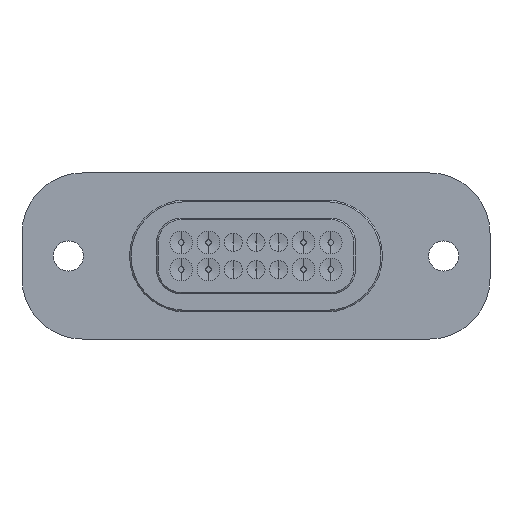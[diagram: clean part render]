
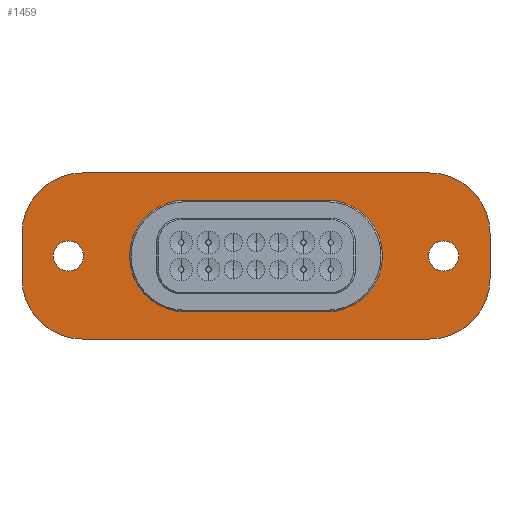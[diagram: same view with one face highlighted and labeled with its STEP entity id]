
A CAD part, front view. The second image highlights one B-rep face of the part: STEP entity #1459.
In plain terms, the highlighted planar face has unit normal (0, -1, 0).
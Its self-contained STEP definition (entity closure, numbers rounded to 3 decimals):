
#57 = DIRECTION ( 'NONE',  ( 0., 0., 1. ) ) ;
#124 = VERTEX_POINT ( 'NONE', #1518 ) ;
#156 = ORIENTED_EDGE ( 'NONE', *, *, #4023, .T. ) ;
#201 = CARTESIAN_POINT ( 'NONE',  ( 11.5, 0., 5.5 ) ) ;
#262 = DIRECTION ( 'NONE',  ( 0., 0., 1. ) ) ;
#278 = AXIS2_PLACEMENT_3D ( 'NONE', #2399, #5189, #822 ) ;
#284 = CARTESIAN_POINT ( 'NONE',  ( -15.5, 0., 1.5 ) ) ;
#300 = LINE ( 'NONE', #991, #3180 ) ;
#317 = EDGE_CURVE ( 'NONE', #6660, #124, #6042, .T. ) ;
#331 = VERTEX_POINT ( 'NONE', #3552 ) ;
#340 = EDGE_CURVE ( 'NONE', #4793, #2393, #2925, .T. ) ;
#360 = ORIENTED_EDGE ( 'NONE', *, *, #6810, .F. ) ;
#394 = ORIENTED_EDGE ( 'NONE', *, *, #2515, .F. ) ;
#575 = DIRECTION ( 'NONE',  ( 0., 0., 1. ) ) ;
#579 = CARTESIAN_POINT ( 'NONE',  ( 12.425, 0., -1. ) ) ;
#596 = DIRECTION ( 'NONE',  ( 0., 1., 0. ) ) ;
#610 = CIRCLE ( 'NONE', #1866, 4. ) ;
#712 = DIRECTION ( 'NONE',  ( 0., 0., -1. ) ) ;
#732 = DIRECTION ( 'NONE',  ( 1., 0., 0. ) ) ;
#759 = CARTESIAN_POINT ( 'NONE',  ( -4.675, 0., -3.7 ) ) ;
#817 = AXIS2_PLACEMENT_3D ( 'NONE', #6340, #1377, #262 ) ;
#818 = AXIS2_PLACEMENT_3D ( 'NONE', #2684, #4881, #575 ) ;
#822 = DIRECTION ( 'NONE',  ( 0., 0., 1. ) ) ;
#828 = EDGE_CURVE ( 'NONE', #3675, #5938, #7060, .T. ) ;
#859 = EDGE_CURVE ( 'NONE', #4183, #4793, #2325, .T. ) ;
#927 = ORIENTED_EDGE ( 'NONE', *, *, #3309, .F. ) ;
#945 = VERTEX_POINT ( 'NONE', #201 ) ;
#991 = CARTESIAN_POINT ( 'NONE',  ( -4.675, 0., 3.7 ) ) ;
#1001 = CARTESIAN_POINT ( 'NONE',  ( 4.675, 0., -3.7 ) ) ;
#1106 = DIRECTION ( 'NONE',  ( 0., -1., 0. ) ) ;
#1184 = VECTOR ( 'NONE', #2231, 1000. ) ;
#1231 = FACE_OUTER_BOUND ( 'NONE', #4790, .T. ) ;
#1261 = AXIS2_PLACEMENT_3D ( 'NONE', #5652, #4681, #5688 ) ;
#1334 = CARTESIAN_POINT ( 'NONE',  ( -15.5, 0., -1.5 ) ) ;
#1377 = DIRECTION ( 'NONE',  ( 0., -1., 0. ) ) ;
#1415 = ORIENTED_EDGE ( 'NONE', *, *, #2551, .F. ) ;
#1459 = ADVANCED_FACE ( 'NONE', ( #2762, #1695, #1231, #4932 ), #6038, .F. ) ;
#1518 = CARTESIAN_POINT ( 'NONE',  ( 12.425, 0., 1. ) ) ;
#1569 = VERTEX_POINT ( 'NONE', #3232 ) ;
#1596 = CIRCLE ( 'NONE', #1261, 4. ) ;
#1614 = CARTESIAN_POINT ( 'NONE',  ( -11.5, 0., 5.5 ) ) ;
#1695 = FACE_BOUND ( 'NONE', #6171, .T. ) ;
#1731 = DIRECTION ( 'NONE',  ( 0., 1., 0. ) ) ;
#1766 = ORIENTED_EDGE ( 'NONE', *, *, #3381, .F. ) ;
#1862 = ORIENTED_EDGE ( 'NONE', *, *, #6662, .F. ) ;
#1866 = AXIS2_PLACEMENT_3D ( 'NONE', #6739, #5154, #3391 ) ;
#1937 = CARTESIAN_POINT ( 'NONE',  ( -11.5, 0., 5.5 ) ) ;
#2052 = ORIENTED_EDGE ( 'NONE', *, *, #6228, .F. ) ;
#2111 = DIRECTION ( 'NONE',  ( -1., 0., 0. ) ) ;
#2172 = AXIS2_PLACEMENT_3D ( 'NONE', #6624, #1731, #2983 ) ;
#2215 = VECTOR ( 'NONE', #2111, 1000. ) ;
#2231 = DIRECTION ( 'NONE',  ( 0., 0., 1. ) ) ;
#2275 = CARTESIAN_POINT ( 'NONE',  ( -15.5, 0., -1.5 ) ) ;
#2325 = CIRCLE ( 'NONE', #5071, 3.7 ) ;
#2327 = CARTESIAN_POINT ( 'NONE',  ( 15.5, 0., 1.5 ) ) ;
#2393 = VERTEX_POINT ( 'NONE', #1001 ) ;
#2399 = CARTESIAN_POINT ( 'NONE',  ( 12.425, 0., 0. ) ) ;
#2489 = DIRECTION ( 'NONE',  ( 0., -1., 0. ) ) ;
#2515 = EDGE_CURVE ( 'NONE', #945, #3675, #7050, .T. ) ;
#2551 = EDGE_CURVE ( 'NONE', #6208, #6693, #610, .T. ) ;
#2578 = EDGE_LOOP ( 'NONE', ( #360, #6477 ) ) ;
#2632 = ORIENTED_EDGE ( 'NONE', *, *, #859, .F. ) ;
#2638 = VECTOR ( 'NONE', #2963, 1000. ) ;
#2660 = ORIENTED_EDGE ( 'NONE', *, *, #6914, .T. ) ;
#2684 = CARTESIAN_POINT ( 'NONE',  ( -12.425, 0., 0. ) ) ;
#2745 = DIRECTION ( 'NONE',  ( 0., 0., 1. ) ) ;
#2762 = FACE_BOUND ( 'NONE', #2578, .T. ) ;
#2779 = CARTESIAN_POINT ( 'NONE',  ( -4.675, 0., 3.7 ) ) ;
#2925 = LINE ( 'NONE', #6197, #2638 ) ;
#2963 = DIRECTION ( 'NONE',  ( 1., 0., 0. ) ) ;
#2983 = DIRECTION ( 'NONE',  ( 0., 0., 1. ) ) ;
#2987 = DIRECTION ( 'NONE',  ( 0., 0., -1. ) ) ;
#3180 = VECTOR ( 'NONE', #5865, 1000. ) ;
#3190 = DIRECTION ( 'NONE',  ( 0., 0., 1. ) ) ;
#3232 = CARTESIAN_POINT ( 'NONE',  ( -12.425, 0., -1. ) ) ;
#3309 = EDGE_CURVE ( 'NONE', #5938, #5661, #1596, .T. ) ;
#3373 = AXIS2_PLACEMENT_3D ( 'NONE', #5493, #596, #57 ) ;
#3381 = EDGE_CURVE ( 'NONE', #6693, #945, #6826, .T. ) ;
#3391 = DIRECTION ( 'NONE',  ( 0., 0., 1. ) ) ;
#3552 = CARTESIAN_POINT ( 'NONE',  ( -11.5, 0., -5.5 ) ) ;
#3675 = VERTEX_POINT ( 'NONE', #2327 ) ;
#3714 = DIRECTION ( 'NONE',  ( 0., 1., 0. ) ) ;
#3847 = CIRCLE ( 'NONE', #4437, 4. ) ;
#3955 = CIRCLE ( 'NONE', #3373, 1. ) ;
#4004 = ORIENTED_EDGE ( 'NONE', *, *, #5084, .F. ) ;
#4005 = VECTOR ( 'NONE', #732, 1000. ) ;
#4023 = EDGE_CURVE ( 'NONE', #4479, #1569, #6521, .T. ) ;
#4071 = CIRCLE ( 'NONE', #4528, 3.7 ) ;
#4183 = VERTEX_POINT ( 'NONE', #2779 ) ;
#4277 = EDGE_CURVE ( 'NONE', #331, #5923, #3847, .T. ) ;
#4423 = EDGE_CURVE ( 'NONE', #6674, #4183, #300, .T. ) ;
#4437 = AXIS2_PLACEMENT_3D ( 'NONE', #6427, #3714, #3190 ) ;
#4479 = VERTEX_POINT ( 'NONE', #6463 ) ;
#4527 = CIRCLE ( 'NONE', #278, 1. ) ;
#4528 = AXIS2_PLACEMENT_3D ( 'NONE', #5139, #2489, #2987 ) ;
#4681 = DIRECTION ( 'NONE',  ( 0., 1., 0. ) ) ;
#4790 = EDGE_LOOP ( 'NONE', ( #1415, #2052, #6040, #1862, #927, #5362, #394, #1766 ) ) ;
#4793 = VERTEX_POINT ( 'NONE', #759 ) ;
#4881 = DIRECTION ( 'NONE',  ( 0., 1., 0. ) ) ;
#4932 = FACE_BOUND ( 'NONE', #5903, .T. ) ;
#4979 = DIRECTION ( 'NONE',  ( 0., 0., -1. ) ) ;
#5004 = LINE ( 'NONE', #2275, #1184 ) ;
#5071 = AXIS2_PLACEMENT_3D ( 'NONE', #5978, #1106, #2745 ) ;
#5084 = EDGE_CURVE ( 'NONE', #2393, #6674, #4071, .T. ) ;
#5139 = CARTESIAN_POINT ( 'NONE',  ( 4.675, 0., 0. ) ) ;
#5154 = DIRECTION ( 'NONE',  ( 0., 1., 0. ) ) ;
#5189 = DIRECTION ( 'NONE',  ( 0., -1., 0. ) ) ;
#5362 = ORIENTED_EDGE ( 'NONE', *, *, #828, .F. ) ;
#5478 = CARTESIAN_POINT ( 'NONE',  ( 4.675, 0., 3.7 ) ) ;
#5493 = CARTESIAN_POINT ( 'NONE',  ( -12.425, 0., 0. ) ) ;
#5652 = CARTESIAN_POINT ( 'NONE',  ( 11.5, 0., -1.5 ) ) ;
#5661 = VERTEX_POINT ( 'NONE', #7011 ) ;
#5688 = DIRECTION ( 'NONE',  ( 0., 0., 1. ) ) ;
#5800 = ORIENTED_EDGE ( 'NONE', *, *, #340, .F. ) ;
#5865 = DIRECTION ( 'NONE',  ( -1., 0., 0. ) ) ;
#5903 = EDGE_LOOP ( 'NONE', ( #4004, #5800, #2632, #6078 ) ) ;
#5923 = VERTEX_POINT ( 'NONE', #1334 ) ;
#5938 = VERTEX_POINT ( 'NONE', #6491 ) ;
#5978 = CARTESIAN_POINT ( 'NONE',  ( -4.675, 0., 0. ) ) ;
#6038 = PLANE ( 'NONE',  #2172 ) ;
#6040 = ORIENTED_EDGE ( 'NONE', *, *, #4277, .F. ) ;
#6042 = CIRCLE ( 'NONE', #817, 1. ) ;
#6057 = CARTESIAN_POINT ( 'NONE',  ( 11.5, 0., 1.5 ) ) ;
#6078 = ORIENTED_EDGE ( 'NONE', *, *, #4423, .F. ) ;
#6171 = EDGE_LOOP ( 'NONE', ( #156, #2660 ) ) ;
#6197 = CARTESIAN_POINT ( 'NONE',  ( -4.675, 0., -3.7 ) ) ;
#6208 = VERTEX_POINT ( 'NONE', #284 ) ;
#6224 = VECTOR ( 'NONE', #4979, 1000. ) ;
#6228 = EDGE_CURVE ( 'NONE', #5923, #6208, #5004, .T. ) ;
#6340 = CARTESIAN_POINT ( 'NONE',  ( 12.425, 0., 0. ) ) ;
#6427 = CARTESIAN_POINT ( 'NONE',  ( -11.5, 0., -1.5 ) ) ;
#6463 = CARTESIAN_POINT ( 'NONE',  ( -12.425, 0., 1. ) ) ;
#6477 = ORIENTED_EDGE ( 'NONE', *, *, #317, .F. ) ;
#6491 = CARTESIAN_POINT ( 'NONE',  ( 15.5, 0., -1.5 ) ) ;
#6519 = CARTESIAN_POINT ( 'NONE',  ( -11.5, 0., -5.5 ) ) ;
#6521 = CIRCLE ( 'NONE', #818, 1. ) ;
#6583 = LINE ( 'NONE', #6519, #2215 ) ;
#6624 = CARTESIAN_POINT ( 'NONE',  ( -11.5, 0., 1.5 ) ) ;
#6660 = VERTEX_POINT ( 'NONE', #579 ) ;
#6662 = EDGE_CURVE ( 'NONE', #5661, #331, #6583, .T. ) ;
#6674 = VERTEX_POINT ( 'NONE', #5478 ) ;
#6678 = DIRECTION ( 'NONE',  ( 0., 1., 0. ) ) ;
#6693 = VERTEX_POINT ( 'NONE', #1614 ) ;
#6739 = CARTESIAN_POINT ( 'NONE',  ( -11.5, 0., 1.5 ) ) ;
#6810 = EDGE_CURVE ( 'NONE', #124, #6660, #4527, .T. ) ;
#6818 = AXIS2_PLACEMENT_3D ( 'NONE', #6057, #6678, #712 ) ;
#6826 = LINE ( 'NONE', #1937, #4005 ) ;
#6914 = EDGE_CURVE ( 'NONE', #1569, #4479, #3955, .T. ) ;
#7011 = CARTESIAN_POINT ( 'NONE',  ( 11.5, 0., -5.5 ) ) ;
#7021 = CARTESIAN_POINT ( 'NONE',  ( 15.5, 0., -1.5 ) ) ;
#7050 = CIRCLE ( 'NONE', #6818, 4. ) ;
#7060 = LINE ( 'NONE', #7021, #6224 ) ;
